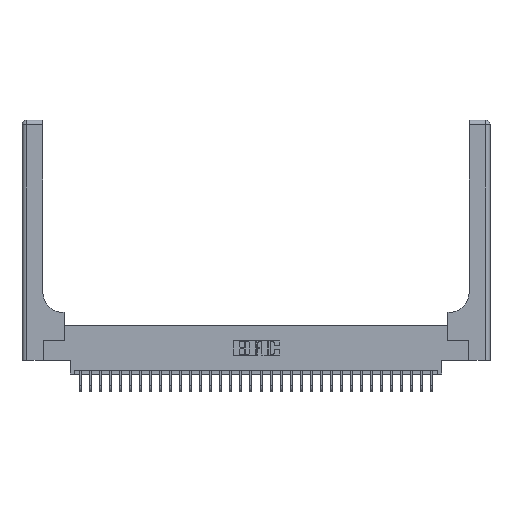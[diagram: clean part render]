
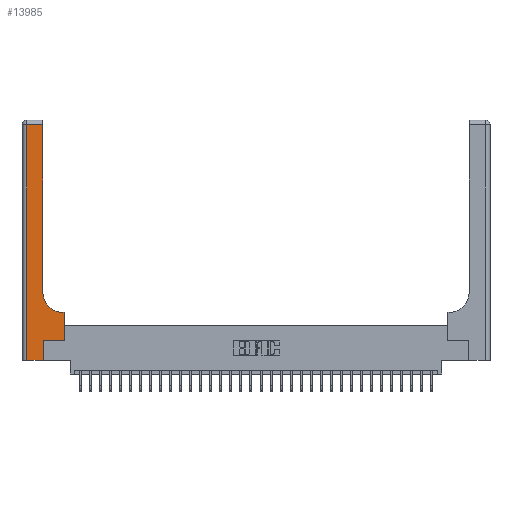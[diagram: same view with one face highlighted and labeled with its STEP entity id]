
A CAD part, top view. The second image highlights one B-rep face of the part: STEP entity #13985.
In plain terms, the highlighted planar face has unit normal (0, 0, 1).
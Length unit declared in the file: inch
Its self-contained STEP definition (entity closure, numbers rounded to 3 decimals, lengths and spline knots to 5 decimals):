
#127 = VECTOR ( 'NONE', #3693, 39.37008 ) ;
#405 = EDGE_CURVE ( 'NONE', #3170, #4683, #18560, .T. ) ;
#602 = CARTESIAN_POINT ( 'NONE',  ( 0., 2.94, 0.37 ) ) ;
#722 = VERTEX_POINT ( 'NONE', #14670 ) ;
#1576 = ORIENTED_EDGE ( 'NONE', *, *, #15285, .T. ) ;
#1676 = DIRECTION ( 'NONE',  ( -1., 0., 0. ) ) ;
#1730 = CARTESIAN_POINT ( 'NONE',  ( 0.06, 0., 0.37 ) ) ;
#1857 = VERTEX_POINT ( 'NONE', #16318 ) ;
#2741 = EDGE_LOOP ( 'NONE', ( #15995, #1576, #8497, #10474, #8230, #16559, #31254, #13213, #23403 ) ) ;
#3170 = VERTEX_POINT ( 'NONE', #30887 ) ;
#3313 = DIRECTION ( 'NONE',  ( 0., 0., -1. ) ) ;
#3693 = DIRECTION ( 'NONE',  ( 0., 1., 0. ) ) ;
#4683 = VERTEX_POINT ( 'NONE', #10186 ) ;
#6487 = CARTESIAN_POINT ( 'NONE',  ( 0.06, 3., 0.37 ) ) ;
#6739 = CARTESIAN_POINT ( 'NONE',  ( 0.528, 0.25, 0.37 ) ) ;
#6917 = EDGE_CURVE ( 'NONE', #4683, #23279, #11274, .T. ) ;
#7420 = EDGE_CURVE ( 'NONE', #10799, #1857, #21807, .T. ) ;
#7461 = VECTOR ( 'NONE', #14367, 39.37008 ) ;
#8230 = ORIENTED_EDGE ( 'NONE', *, *, #8333, .T. ) ;
#8333 = EDGE_CURVE ( 'NONE', #26160, #3170, #26808, .T. ) ;
#8497 = ORIENTED_EDGE ( 'NONE', *, *, #14560, .T. ) ;
#9001 = VECTOR ( 'NONE', #20445, 39.37008 ) ;
#9351 = DIRECTION ( 'NONE',  ( 0., 1., 0. ) ) ;
#9743 = VECTOR ( 'NONE', #20348, 39.37008 ) ;
#10186 = CARTESIAN_POINT ( 'NONE',  ( 0.528, 0.25, 0.37 ) ) ;
#10474 = ORIENTED_EDGE ( 'NONE', *, *, #18739, .T. ) ;
#10799 = VERTEX_POINT ( 'NONE', #13074 ) ;
#10874 = FACE_OUTER_BOUND ( 'NONE', #2741, .T. ) ;
#11274 = LINE ( 'NONE', #6739, #127 ) ;
#12497 = VECTOR ( 'NONE', #16462, 39.37008 ) ;
#13074 = CARTESIAN_POINT ( 'NONE',  ( 0.51, 0.6, 0.37 ) ) ;
#13213 = ORIENTED_EDGE ( 'NONE', *, *, #14082, .T. ) ;
#13325 = VERTEX_POINT ( 'NONE', #29224 ) ;
#13899 = CARTESIAN_POINT ( 'NONE',  ( 0.26, 3., 0.37 ) ) ;
#13932 = LINE ( 'NONE', #21678, #20988 ) ;
#13985 = ADVANCED_FACE ( 'NONE', ( #10874 ), #15555, .F. ) ;
#14031 = LINE ( 'NONE', #17086, #12497 ) ;
#14082 = EDGE_CURVE ( 'NONE', #23279, #10799, #13932, .T. ) ;
#14133 = DIRECTION ( 'NONE',  ( 1., 0., 0. ) ) ;
#14367 = DIRECTION ( 'NONE',  ( 0., -1., 0. ) ) ;
#14436 = EDGE_CURVE ( 'NONE', #1857, #722, #30522, .T. ) ;
#14511 = CARTESIAN_POINT ( 'NONE',  ( 0.265, 0., 0.37 ) ) ;
#14560 = EDGE_CURVE ( 'NONE', #13325, #27087, #21323, .T. ) ;
#14670 = CARTESIAN_POINT ( 'NONE',  ( 0.26, 2.94, 0.37 ) ) ;
#15285 = EDGE_CURVE ( 'NONE', #722, #13325, #22706, .T. ) ;
#15555 = PLANE ( 'NONE',  #30778 ) ;
#15995 = ORIENTED_EDGE ( 'NONE', *, *, #14436, .T. ) ;
#16318 = CARTESIAN_POINT ( 'NONE',  ( 0.26, 0.85, 0.37 ) ) ;
#16462 = DIRECTION ( 'NONE',  ( 1., 0., 0. ) ) ;
#16479 = DIRECTION ( 'NONE',  ( 0., 1., 0. ) ) ;
#16559 = ORIENTED_EDGE ( 'NONE', *, *, #405, .T. ) ;
#17086 = CARTESIAN_POINT ( 'NONE',  ( 0., 0., 0.37 ) ) ;
#18230 = VECTOR ( 'NONE', #9351, 39.37008 ) ;
#18239 = CARTESIAN_POINT ( 'NONE',  ( 0.528, 0.6, 0.37 ) ) ;
#18560 = LINE ( 'NONE', #25837, #9743 ) ;
#18739 = EDGE_CURVE ( 'NONE', #27087, #26160, #14031, .T. ) ;
#20348 = DIRECTION ( 'NONE',  ( 1., 0., 0. ) ) ;
#20445 = DIRECTION ( 'NONE',  ( -1., 0., 0. ) ) ;
#20717 = DIRECTION ( 'NONE',  ( -1., 0., 0. ) ) ;
#20988 = VECTOR ( 'NONE', #1676, 39.37008 ) ;
#21323 = LINE ( 'NONE', #6487, #7461 ) ;
#21678 = CARTESIAN_POINT ( 'NONE',  ( 0.26, 0.6, 0.37 ) ) ;
#21807 = CIRCLE ( 'NONE', #30051, 0.25 ) ;
#22706 = LINE ( 'NONE', #602, #9001 ) ;
#23279 = VERTEX_POINT ( 'NONE', #18239 ) ;
#23403 = ORIENTED_EDGE ( 'NONE', *, *, #7420, .T. ) ;
#24086 = CARTESIAN_POINT ( 'NONE',  ( 0.265, 0., 0.37 ) ) ;
#25404 = CARTESIAN_POINT ( 'NONE',  ( 0., 3., 0.37 ) ) ;
#25837 = CARTESIAN_POINT ( 'NONE',  ( 0.265, 0.25, 0.37 ) ) ;
#26104 = CARTESIAN_POINT ( 'NONE',  ( 0.51, 0.85, 0.37 ) ) ;
#26160 = VERTEX_POINT ( 'NONE', #24086 ) ;
#26808 = LINE ( 'NONE', #14511, #18230 ) ;
#27087 = VERTEX_POINT ( 'NONE', #1730 ) ;
#28103 = VECTOR ( 'NONE', #16479, 39.37008 ) ;
#29224 = CARTESIAN_POINT ( 'NONE',  ( 0.06, 2.94, 0.37 ) ) ;
#30051 = AXIS2_PLACEMENT_3D ( 'NONE', #26104, #30918, #14133 ) ;
#30522 = LINE ( 'NONE', #13899, #28103 ) ;
#30778 = AXIS2_PLACEMENT_3D ( 'NONE', #25404, #3313, #20717 ) ;
#30887 = CARTESIAN_POINT ( 'NONE',  ( 0.265, 0.25, 0.37 ) ) ;
#30918 = DIRECTION ( 'NONE',  ( 0., 0., -1. ) ) ;
#31254 = ORIENTED_EDGE ( 'NONE', *, *, #6917, .T. ) ;
